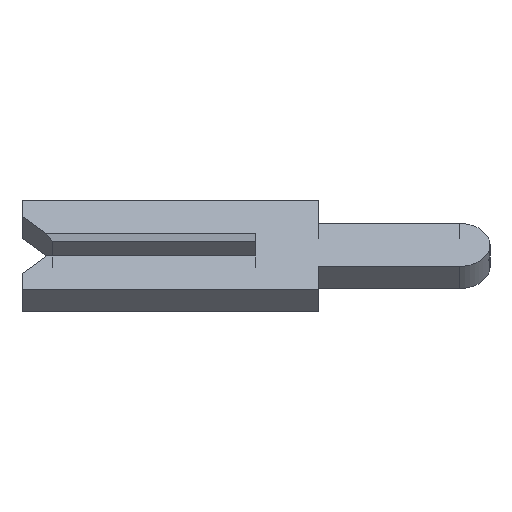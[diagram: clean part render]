
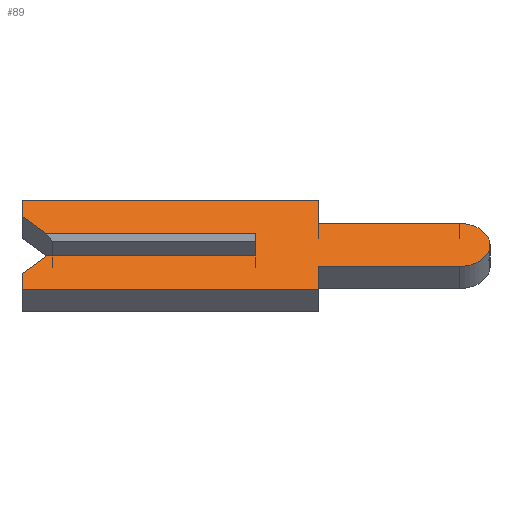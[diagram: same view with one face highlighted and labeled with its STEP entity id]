
A CAD part, left-side view. The second image highlights one B-rep face of the part: STEP entity #89.
In plain terms, the highlighted face is planar.
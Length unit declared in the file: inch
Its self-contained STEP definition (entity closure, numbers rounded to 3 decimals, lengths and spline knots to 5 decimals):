
#6 = CARTESIAN_POINT ( 'NONE',  ( -0.01, 0.15, 0.04 ) ) ;
#33 = ORIENTED_EDGE ( 'NONE', *, *, #1121, .F. ) ;
#76 = LINE ( 'NONE', #1728, #1295 ) ;
#78 = FACE_OUTER_BOUND ( 'NONE', #817, .T. ) ;
#89 = ADVANCED_FACE ( 'NONE', ( #78 ), #136, .F. ) ;
#92 = EDGE_CURVE ( 'NONE', #1743, #724, #1564, .T. ) ;
#101 = ORIENTED_EDGE ( 'NONE', *, *, #669, .F. ) ;
#105 = VECTOR ( 'NONE', #494, 39.37008 ) ;
#129 = LINE ( 'NONE', #2304, #821 ) ;
#136 = PLANE ( 'NONE',  #2320 ) ;
#153 = ORIENTED_EDGE ( 'NONE', *, *, #906, .F. ) ;
#187 = LINE ( 'NONE', #1409, #275 ) ;
#192 = DIRECTION ( 'NONE',  ( 0., -1., 0. ) ) ;
#215 = CARTESIAN_POINT ( 'NONE',  ( -0.01, -0.04, 0.04 ) ) ;
#237 = ORIENTED_EDGE ( 'NONE', *, *, #951, .F. ) ;
#247 = LINE ( 'NONE', #273, #1419 ) ;
#273 = CARTESIAN_POINT ( 'NONE',  ( -0.01, 0.1305, -0.0065 ) ) ;
#275 = VECTOR ( 'NONE', #2316, 39.37008 ) ;
#276 = ORIENTED_EDGE ( 'NONE', *, *, #1015, .T. ) ;
#311 = CARTESIAN_POINT ( 'NONE',  ( -0.01, -0.04, -0.0195 ) ) ;
#333 = LINE ( 'NONE', #1737, #761 ) ;
#337 = CARTESIAN_POINT ( 'NONE',  ( -0.01, -0.04, 0.0195 ) ) ;
#368 = LINE ( 'NONE', #2098, #2169 ) ;
#393 = CARTESIAN_POINT ( 'NONE',  ( -0.01, 0.15, -0.026 ) ) ;
#424 = ORIENTED_EDGE ( 'NONE', *, *, #1286, .F. ) ;
#440 = CARTESIAN_POINT ( 'NONE',  ( -0.01, 0.134, 0.01 ) ) ;
#494 = DIRECTION ( 'NONE',  ( 0., 1., 0. ) ) ;
#504 = ORIENTED_EDGE ( 'NONE', *, *, #1338, .F. ) ;
#509 = DIRECTION ( 'NONE',  ( 1., 0., 0. ) ) ;
#523 = CARTESIAN_POINT ( 'NONE',  ( -0.01, -0.1305, 0. ) ) ;
#605 = DIRECTION ( 'NONE',  ( 0., -1., 0. ) ) ;
#615 = CARTESIAN_POINT ( 'NONE',  ( -0.01, -0.1305, 0. ) ) ;
#637 = CARTESIAN_POINT ( 'NONE',  ( -0.01, -0.1305, -0.0195 ) ) ;
#669 = EDGE_CURVE ( 'NONE', #1468, #1841, #1937, .T. ) ;
#677 = DIRECTION ( 'NONE',  ( 0., 0., 1. ) ) ;
#724 = VERTEX_POINT ( 'NONE', #2111 ) ;
#745 = EDGE_CURVE ( 'NONE', #1067, #1468, #969, .T. ) ;
#757 = CARTESIAN_POINT ( 'NONE',  ( -0.01, -0.04, 0.0195 ) ) ;
#761 = VECTOR ( 'NONE', #605, 39.37008 ) ;
#783 = VERTEX_POINT ( 'NONE', #6 ) ;
#787 = ORIENTED_EDGE ( 'NONE', *, *, #1467, .F. ) ;
#792 = CARTESIAN_POINT ( 'NONE',  ( -0.01, 0.15, 0.026 ) ) ;
#817 = EDGE_LOOP ( 'NONE', ( #276, #424, #33, #1999, #1511, #237, #504, #1341, #1197, #101, #1474, #1713, #153, #787 ) ) ;
#821 = VECTOR ( 'NONE', #677, 39.37008 ) ;
#849 = LINE ( 'NONE', #1000, #2227 ) ;
#852 = LINE ( 'NONE', #792, #2170 ) ;
#906 = EDGE_CURVE ( 'NONE', #1294, #783, #852, .T. ) ;
#910 = VECTOR ( 'NONE', #2088, 39.37008 ) ;
#951 = EDGE_CURVE ( 'NONE', #1820, #2062, #76, .T. ) ;
#967 = LINE ( 'NONE', #2337, #1361 ) ;
#969 = LINE ( 'NONE', #1888, #910 ) ;
#994 = DIRECTION ( 'NONE',  ( 0., 0., -1. ) ) ;
#1000 = CARTESIAN_POINT ( 'NONE',  ( -0.01, 0.1305, 0.0065 ) ) ;
#1015 = EDGE_CURVE ( 'NONE', #1582, #1927, #368, .T. ) ;
#1032 = CARTESIAN_POINT ( 'NONE',  ( -0.01, 0., -0.01 ) ) ;
#1046 = VERTEX_POINT ( 'NONE', #393 ) ;
#1061 = CARTESIAN_POINT ( 'NONE',  ( -0.01, -0.04, -0.04 ) ) ;
#1067 = VERTEX_POINT ( 'NONE', #215 ) ;
#1121 = EDGE_CURVE ( 'NONE', #2035, #1959, #333, .T. ) ;
#1128 = DIRECTION ( 'NONE',  ( 0., -1., 0. ) ) ;
#1150 = DIRECTION ( 'NONE',  ( 0., 1., 0. ) ) ;
#1192 = DIRECTION ( 'NONE',  ( 0., 0.707, 0.707 ) ) ;
#1197 = ORIENTED_EDGE ( 'NONE', *, *, #1632, .F. ) ;
#1286 = EDGE_CURVE ( 'NONE', #1959, #1927, #187, .T. ) ;
#1294 = VERTEX_POINT ( 'NONE', #2126 ) ;
#1295 = VECTOR ( 'NONE', #1150, 39.37008 ) ;
#1338 = EDGE_CURVE ( 'NONE', #724, #1820, #967, .T. ) ;
#1341 = ORIENTED_EDGE ( 'NONE', *, *, #92, .F. ) ;
#1361 = VECTOR ( 'NONE', #1744, 39.37008 ) ;
#1369 = DIRECTION ( 'NONE',  ( 0., 0., 1. ) ) ;
#1371 = EDGE_CURVE ( 'NONE', #783, #1067, #2315, .T. ) ;
#1409 = CARTESIAN_POINT ( 'NONE',  ( -0.01, 0., 0.0065 ) ) ;
#1416 = VECTOR ( 'NONE', #1128, 39.37008 ) ;
#1419 = VECTOR ( 'NONE', #1607, 39.37008 ) ;
#1467 = EDGE_CURVE ( 'NONE', #1582, #1294, #849, .T. ) ;
#1468 = VERTEX_POINT ( 'NONE', #337 ) ;
#1474 = ORIENTED_EDGE ( 'NONE', *, *, #745, .F. ) ;
#1511 = ORIENTED_EDGE ( 'NONE', *, *, #1828, .F. ) ;
#1564 = LINE ( 'NONE', #311, #105 ) ;
#1582 = VERTEX_POINT ( 'NONE', #440 ) ;
#1607 = DIRECTION ( 'NONE',  ( 0., -0.707, 0.707 ) ) ;
#1626 = CARTESIAN_POINT ( 'NONE',  ( -0.01, 0.15, -0.04 ) ) ;
#1632 = EDGE_CURVE ( 'NONE', #1841, #1743, #2343, .T. ) ;
#1670 = VECTOR ( 'NONE', #2029, 39.37008 ) ;
#1713 = ORIENTED_EDGE ( 'NONE', *, *, #1371, .F. ) ;
#1728 = CARTESIAN_POINT ( 'NONE',  ( -0.01, 0.15, -0.04 ) ) ;
#1737 = CARTESIAN_POINT ( 'NONE',  ( -0.01, -0.1305, -0.01 ) ) ;
#1743 = VERTEX_POINT ( 'NONE', #637 ) ;
#1744 = DIRECTION ( 'NONE',  ( 0., 0., -1. ) ) ;
#1820 = VERTEX_POINT ( 'NONE', #1061 ) ;
#1828 = EDGE_CURVE ( 'NONE', #2062, #1046, #129, .T. ) ;
#1841 = VERTEX_POINT ( 'NONE', #1990 ) ;
#1888 = CARTESIAN_POINT ( 'NONE',  ( -0.01, -0.04, 0.04 ) ) ;
#1927 = VERTEX_POINT ( 'NONE', #2353 ) ;
#1932 = AXIS2_PLACEMENT_3D ( 'NONE', #615, #1939, #994 ) ;
#1937 = LINE ( 'NONE', #757, #1670 ) ;
#1939 = DIRECTION ( 'NONE',  ( 1., 0., 0. ) ) ;
#1959 = VERTEX_POINT ( 'NONE', #1032 ) ;
#1990 = CARTESIAN_POINT ( 'NONE',  ( -0.01, -0.1305, 0.0195 ) ) ;
#1998 = DIRECTION ( 'NONE',  ( 0., 0., -1. ) ) ;
#1999 = ORIENTED_EDGE ( 'NONE', *, *, #2204, .F. ) ;
#2029 = DIRECTION ( 'NONE',  ( 0., -1., 0. ) ) ;
#2035 = VERTEX_POINT ( 'NONE', #2361 ) ;
#2062 = VERTEX_POINT ( 'NONE', #1626 ) ;
#2088 = DIRECTION ( 'NONE',  ( 0., 0., -1. ) ) ;
#2098 = CARTESIAN_POINT ( 'NONE',  ( -0.01, 0.15, 0.01 ) ) ;
#2111 = CARTESIAN_POINT ( 'NONE',  ( -0.01, -0.04, -0.0195 ) ) ;
#2126 = CARTESIAN_POINT ( 'NONE',  ( -0.01, 0.15, 0.026 ) ) ;
#2169 = VECTOR ( 'NONE', #192, 39.37008 ) ;
#2170 = VECTOR ( 'NONE', #1369, 39.37008 ) ;
#2195 = CARTESIAN_POINT ( 'NONE',  ( -0.01, 0.15, 0.04 ) ) ;
#2204 = EDGE_CURVE ( 'NONE', #1046, #2035, #247, .T. ) ;
#2227 = VECTOR ( 'NONE', #1192, 39.37008 ) ;
#2304 = CARTESIAN_POINT ( 'NONE',  ( -0.01, 0.15, -0.026 ) ) ;
#2315 = LINE ( 'NONE', #2195, #1416 ) ;
#2316 = DIRECTION ( 'NONE',  ( 0., 0., 1. ) ) ;
#2320 = AXIS2_PLACEMENT_3D ( 'NONE', #523, #509, #1998 ) ;
#2337 = CARTESIAN_POINT ( 'NONE',  ( -0.01, -0.04, -0.04 ) ) ;
#2343 = CIRCLE ( 'NONE', #1932, 0.0195 ) ;
#2353 = CARTESIAN_POINT ( 'NONE',  ( -0.01, 0., 0.01 ) ) ;
#2361 = CARTESIAN_POINT ( 'NONE',  ( -0.01, 0.134, -0.01 ) ) ;
